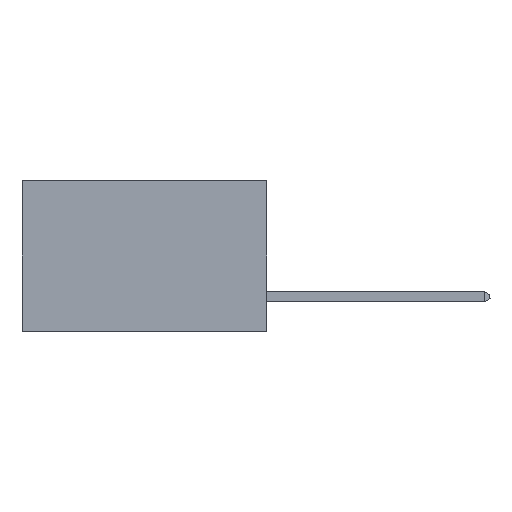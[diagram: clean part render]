
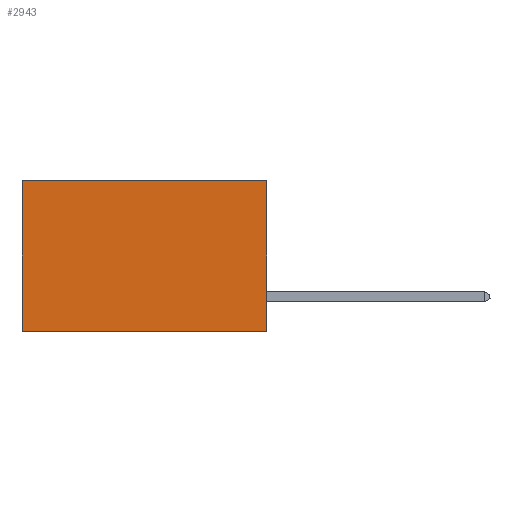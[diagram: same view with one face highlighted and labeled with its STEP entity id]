
A CAD part, left-side view. The second image highlights one B-rep face of the part: STEP entity #2943.
In plain terms, the highlighted planar face has unit normal (-1, 0, 0).
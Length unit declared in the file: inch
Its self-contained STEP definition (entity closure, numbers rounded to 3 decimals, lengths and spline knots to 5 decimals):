
#10 = VECTOR ( 'NONE', #3189, 39.37008 ) ;
#364 = PLANE ( 'NONE',  #10332 ) ;
#756 = VERTEX_POINT ( 'NONE', #8693 ) ;
#1359 = DIRECTION ( 'NONE',  ( 0., 0., -1. ) ) ;
#2934 = LINE ( 'NONE', #3991, #10 ) ;
#2939 = CARTESIAN_POINT ( 'NONE',  ( 0.2875, 0., -0.37 ) ) ;
#2943 = ADVANCED_FACE ( 'NONE', ( #12583 ), #364, .F. ) ;
#3029 = CARTESIAN_POINT ( 'NONE',  ( 0.2875, 0., 0. ) ) ;
#3189 = DIRECTION ( 'NONE',  ( 0., 0., -1. ) ) ;
#3279 = LINE ( 'NONE', #6131, #5277 ) ;
#3501 = EDGE_CURVE ( 'NONE', #4735, #6628, #3279, .T. ) ;
#3991 = CARTESIAN_POINT ( 'NONE',  ( 0.2875, 0.6, 0. ) ) ;
#4241 = ORIENTED_EDGE ( 'NONE', *, *, #3501, .F. ) ;
#4735 = VERTEX_POINT ( 'NONE', #3029 ) ;
#5277 = VECTOR ( 'NONE', #8362, 39.37008 ) ;
#5495 = EDGE_CURVE ( 'NONE', #756, #9015, #2934, .T. ) ;
#5501 = CARTESIAN_POINT ( 'NONE',  ( 0.2875, 0.6, -0.37 ) ) ;
#5903 = LINE ( 'NONE', #7104, #11336 ) ;
#6001 = DIRECTION ( 'NONE',  ( 0., 1., 0. ) ) ;
#6131 = CARTESIAN_POINT ( 'NONE',  ( 0.2875, 0., 0. ) ) ;
#6628 = VERTEX_POINT ( 'NONE', #2939 ) ;
#7104 = CARTESIAN_POINT ( 'NONE',  ( 0.2875, 0., 0. ) ) ;
#7259 = EDGE_LOOP ( 'NONE', ( #11786, #9136, #4241, #7384 ) ) ;
#7287 = CARTESIAN_POINT ( 'NONE',  ( 0.2875, 0., 0. ) ) ;
#7384 = ORIENTED_EDGE ( 'NONE', *, *, #11071, .T. ) ;
#8101 = EDGE_CURVE ( 'NONE', #6628, #9015, #8133, .T. ) ;
#8133 = LINE ( 'NONE', #11631, #11998 ) ;
#8331 = DIRECTION ( 'NONE',  ( 1., 0., 0. ) ) ;
#8362 = DIRECTION ( 'NONE',  ( 0., 0., -1. ) ) ;
#8693 = CARTESIAN_POINT ( 'NONE',  ( 0.2875, 0.6, 0. ) ) ;
#9015 = VERTEX_POINT ( 'NONE', #5501 ) ;
#9136 = ORIENTED_EDGE ( 'NONE', *, *, #8101, .F. ) ;
#10332 = AXIS2_PLACEMENT_3D ( 'NONE', #7287, #8331, #1359 ) ;
#11071 = EDGE_CURVE ( 'NONE', #4735, #756, #5903, .T. ) ;
#11336 = VECTOR ( 'NONE', #6001, 39.37008 ) ;
#11631 = CARTESIAN_POINT ( 'NONE',  ( 0.2875, 0., -0.37 ) ) ;
#11786 = ORIENTED_EDGE ( 'NONE', *, *, #5495, .T. ) ;
#11998 = VECTOR ( 'NONE', #12626, 39.37008 ) ;
#12583 = FACE_OUTER_BOUND ( 'NONE', #7259, .T. ) ;
#12626 = DIRECTION ( 'NONE',  ( 0., 1., 0. ) ) ;
